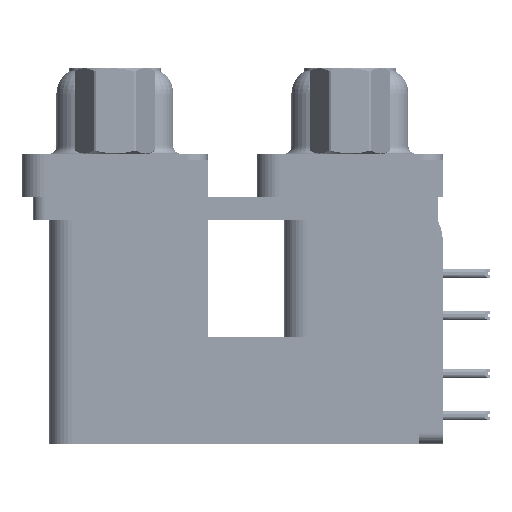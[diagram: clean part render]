
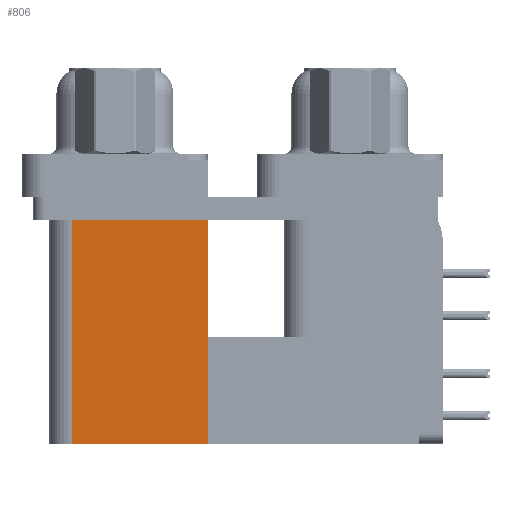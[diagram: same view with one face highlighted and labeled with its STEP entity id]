
A CAD part, left-side view. The second image highlights one B-rep face of the part: STEP entity #806.
In plain terms, the highlighted planar face has unit normal (-1, 0, 0).
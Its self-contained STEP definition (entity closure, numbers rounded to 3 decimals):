
#208 = EDGE_LOOP ( 'NONE', ( #47699, #28721, #2758, #49960 ) ) ;
#535 = DIRECTION ( 'NONE',  ( 0., 1., 0. ) ) ;
#797 = CARTESIAN_POINT ( 'NONE',  ( 3.765, 9.6, -19.2 ) ) ;
#806 = ADVANCED_FACE ( 'NONE', ( #25646 ), #41955, .F. ) ;
#1935 = VECTOR ( 'NONE', #16108, 1000. ) ;
#2323 = VERTEX_POINT ( 'NONE', #53493 ) ;
#2758 = ORIENTED_EDGE ( 'NONE', *, *, #42239, .F. ) ;
#7561 = CARTESIAN_POINT ( 'NONE',  ( 3.765, 18.8, -19.2 ) ) ;
#8619 = CARTESIAN_POINT ( 'NONE',  ( 3.765, 9.6, -2.5 ) ) ;
#9073 = CARTESIAN_POINT ( 'NONE',  ( 3.765, 18.8, -2.5 ) ) ;
#9655 = EDGE_CURVE ( 'NONE', #35444, #42616, #27766, .T. ) ;
#9674 = DIRECTION ( 'NONE',  ( 1., 0., 0. ) ) ;
#15962 = AXIS2_PLACEMENT_3D ( 'NONE', #37869, #9674, #34351 ) ;
#16108 = DIRECTION ( 'NONE',  ( 0., 0., 1. ) ) ;
#16813 = LINE ( 'NONE', #797, #30135 ) ;
#18286 = VERTEX_POINT ( 'NONE', #8619 ) ;
#21942 = CARTESIAN_POINT ( 'NONE',  ( 3.765, 9.6, -19.2 ) ) ;
#25646 = FACE_OUTER_BOUND ( 'NONE', #208, .T. ) ;
#26480 = DIRECTION ( 'NONE',  ( 0., 1., 0. ) ) ;
#27766 = LINE ( 'NONE', #28835, #1935 ) ;
#28721 = ORIENTED_EDGE ( 'NONE', *, *, #9655, .F. ) ;
#28835 = CARTESIAN_POINT ( 'NONE',  ( 3.765, 18.8, -19.2 ) ) ;
#29788 = VECTOR ( 'NONE', #26480, 1000. ) ;
#30135 = VECTOR ( 'NONE', #535, 1000. ) ;
#30630 = LINE ( 'NONE', #21942, #33221 ) ;
#32955 = EDGE_CURVE ( 'NONE', #2323, #18286, #30630, .T. ) ;
#33221 = VECTOR ( 'NONE', #34426, 1000. ) ;
#34115 = CARTESIAN_POINT ( 'NONE',  ( 3.765, 9.6, -2.5 ) ) ;
#34351 = DIRECTION ( 'NONE',  ( 0., 0., -1. ) ) ;
#34426 = DIRECTION ( 'NONE',  ( 0., 0., 1. ) ) ;
#34544 = EDGE_CURVE ( 'NONE', #18286, #42616, #51728, .T. ) ;
#35444 = VERTEX_POINT ( 'NONE', #7561 ) ;
#37869 = CARTESIAN_POINT ( 'NONE',  ( 3.765, 9.6, -19.2 ) ) ;
#41955 = PLANE ( 'NONE',  #15962 ) ;
#42239 = EDGE_CURVE ( 'NONE', #2323, #35444, #16813, .T. ) ;
#42616 = VERTEX_POINT ( 'NONE', #9073 ) ;
#47699 = ORIENTED_EDGE ( 'NONE', *, *, #34544, .T. ) ;
#49960 = ORIENTED_EDGE ( 'NONE', *, *, #32955, .T. ) ;
#51728 = LINE ( 'NONE', #34115, #29788 ) ;
#53493 = CARTESIAN_POINT ( 'NONE',  ( 3.765, 9.6, -19.2 ) ) ;
